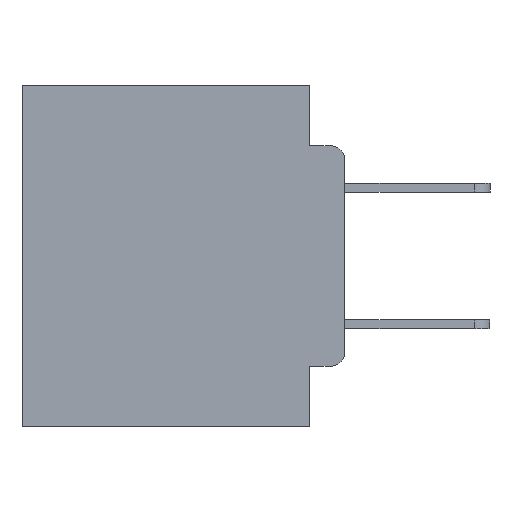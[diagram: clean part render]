
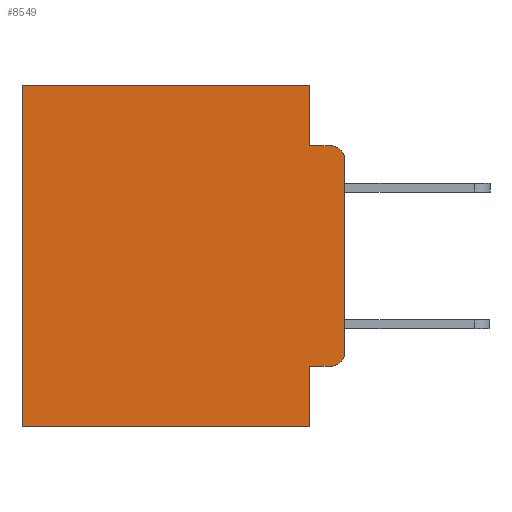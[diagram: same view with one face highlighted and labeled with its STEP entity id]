
A CAD part, left-side view. The second image highlights one B-rep face of the part: STEP entity #8549.
In plain terms, the highlighted planar face has unit normal (-1, 0, 0).
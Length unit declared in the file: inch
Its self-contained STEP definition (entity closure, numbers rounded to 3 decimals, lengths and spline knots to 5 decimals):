
#955 = DIRECTION ( 'NONE',  ( 0., 0., -1. ) ) ;
#1139 = AXIS2_PLACEMENT_3D ( 'NONE', #22405, #25187, #23031 ) ;
#1658 = CARTESIAN_POINT ( 'NONE',  ( 0.298, 0., -0.5 ) ) ;
#1908 = VERTEX_POINT ( 'NONE', #9484 ) ;
#1999 = AXIS2_PLACEMENT_3D ( 'NONE', #7386, #13831, #955 ) ;
#2071 = CARTESIAN_POINT ( 'NONE',  ( 0.298, 0., 0. ) ) ;
#2435 = EDGE_CURVE ( 'NONE', #12989, #2674, #8465, .T. ) ;
#2674 = VERTEX_POINT ( 'NONE', #13288 ) ;
#2750 = VECTOR ( 'NONE', #10493, 39.37008 ) ;
#2887 = ORIENTED_EDGE ( 'NONE', *, *, #24228, .F. ) ;
#3132 = VECTOR ( 'NONE', #14934, 39.37008 ) ;
#3242 = EDGE_CURVE ( 'NONE', #9568, #12023, #23749, .T. ) ;
#3334 = LINE ( 'NONE', #8640, #14666 ) ;
#3702 = ORIENTED_EDGE ( 'NONE', *, *, #3922, .T. ) ;
#3922 = EDGE_CURVE ( 'NONE', #1908, #19624, #14898, .T. ) ;
#3999 = VECTOR ( 'NONE', #18439, 39.37008 ) ;
#6226 = VERTEX_POINT ( 'NONE', #18835 ) ;
#6266 = VECTOR ( 'NONE', #23988, 39.37008 ) ;
#6347 = CARTESIAN_POINT ( 'NONE',  ( 0.298, 0.473, -0.5 ) ) ;
#6814 = CARTESIAN_POINT ( 'NONE',  ( 0.298, 0.051, 0. ) ) ;
#7386 = CARTESIAN_POINT ( 'NONE',  ( 0.298, 0., 0. ) ) ;
#7534 = EDGE_LOOP ( 'NONE', ( #11947, #11253, #23804, #2887, #17305, #3702, #9386, #14583, #17717, #13311 ) ) ;
#8465 = LINE ( 'NONE', #6814, #2750 ) ;
#8549 = ADVANCED_FACE ( 'NONE', ( #11725 ), #20108, .F. ) ;
#8562 = CARTESIAN_POINT ( 'NONE',  ( 0.298, 0., 0. ) ) ;
#8640 = CARTESIAN_POINT ( 'NONE',  ( 0.298, 0.051, -0.4115 ) ) ;
#8849 = LINE ( 'NONE', #1658, #3132 ) ;
#9386 = ORIENTED_EDGE ( 'NONE', *, *, #26459, .F. ) ;
#9436 = AXIS2_PLACEMENT_3D ( 'NONE', #12673, #27219, #14789 ) ;
#9484 = CARTESIAN_POINT ( 'NONE',  ( 0.298, 0.473, 0. ) ) ;
#9568 = VERTEX_POINT ( 'NONE', #25032 ) ;
#10493 = DIRECTION ( 'NONE',  ( 0., 0., -1. ) ) ;
#10741 = CARTESIAN_POINT ( 'NONE',  ( 0.298, 0.473, 0. ) ) ;
#10843 = EDGE_CURVE ( 'NONE', #9568, #13972, #24900, .T. ) ;
#10879 = EDGE_CURVE ( 'NONE', #24064, #1908, #24271, .T. ) ;
#11253 = ORIENTED_EDGE ( 'NONE', *, *, #3242, .T. ) ;
#11314 = LINE ( 'NONE', #11469, #6266 ) ;
#11469 = CARTESIAN_POINT ( 'NONE',  ( 0.298, 0.051, 0. ) ) ;
#11725 = FACE_OUTER_BOUND ( 'NONE', #7534, .T. ) ;
#11947 = ORIENTED_EDGE ( 'NONE', *, *, #10843, .F. ) ;
#12023 = VERTEX_POINT ( 'NONE', #26804 ) ;
#12257 = CIRCLE ( 'NONE', #9436, 0.02 ) ;
#12439 = CARTESIAN_POINT ( 'NONE',  ( 0.298, 0.051, -0.4115 ) ) ;
#12673 = CARTESIAN_POINT ( 'NONE',  ( 0.298, 0.02, -0.3915 ) ) ;
#12989 = VERTEX_POINT ( 'NONE', #12439 ) ;
#13288 = CARTESIAN_POINT ( 'NONE',  ( 0.298, 0.051, -0.5 ) ) ;
#13311 = ORIENTED_EDGE ( 'NONE', *, *, #20097, .T. ) ;
#13826 = VECTOR ( 'NONE', #23273, 39.37008 ) ;
#13831 = DIRECTION ( 'NONE',  ( 1., 0., 0. ) ) ;
#13972 = VERTEX_POINT ( 'NONE', #19870 ) ;
#14583 = ORIENTED_EDGE ( 'NONE', *, *, #2435, .F. ) ;
#14666 = VECTOR ( 'NONE', #25400, 39.37008 ) ;
#14789 = DIRECTION ( 'NONE',  ( 0., 0., -1. ) ) ;
#14898 = LINE ( 'NONE', #10741, #16217 ) ;
#14934 = DIRECTION ( 'NONE',  ( 0., 1., 0. ) ) ;
#16217 = VECTOR ( 'NONE', #17073, 39.37008 ) ;
#16305 = CARTESIAN_POINT ( 'NONE',  ( 0.298, 0.051, -0.0885 ) ) ;
#17073 = DIRECTION ( 'NONE',  ( 0., 0., -1. ) ) ;
#17149 = CARTESIAN_POINT ( 'NONE',  ( 0.298, 0.051, 0. ) ) ;
#17305 = ORIENTED_EDGE ( 'NONE', *, *, #10879, .T. ) ;
#17592 = VERTEX_POINT ( 'NONE', #26124 ) ;
#17717 = ORIENTED_EDGE ( 'NONE', *, *, #22864, .T. ) ;
#18439 = DIRECTION ( 'NONE',  ( 0., -1., 0. ) ) ;
#18776 = VECTOR ( 'NONE', #21323, 39.37008 ) ;
#18835 = CARTESIAN_POINT ( 'NONE',  ( 0.298, 0.02, -0.4115 ) ) ;
#19624 = VERTEX_POINT ( 'NONE', #6347 ) ;
#19870 = CARTESIAN_POINT ( 'NONE',  ( 0.298, 0., -0.3915 ) ) ;
#20097 = EDGE_CURVE ( 'NONE', #6226, #13972, #12257, .T. ) ;
#20108 = PLANE ( 'NONE',  #1999 ) ;
#20271 = LINE ( 'NONE', #16305, #3999 ) ;
#21323 = DIRECTION ( 'NONE',  ( 0., 1., 0. ) ) ;
#22405 = CARTESIAN_POINT ( 'NONE',  ( 0.298, 0.02, -0.1085 ) ) ;
#22864 = EDGE_CURVE ( 'NONE', #12989, #6226, #3334, .T. ) ;
#23031 = DIRECTION ( 'NONE',  ( 0., 0., -1. ) ) ;
#23235 = EDGE_CURVE ( 'NONE', #17592, #12023, #20271, .T. ) ;
#23273 = DIRECTION ( 'NONE',  ( 0., 0., -1. ) ) ;
#23749 = CIRCLE ( 'NONE', #1139, 0.02 ) ;
#23804 = ORIENTED_EDGE ( 'NONE', *, *, #23235, .F. ) ;
#23988 = DIRECTION ( 'NONE',  ( 0., 0., -1. ) ) ;
#24064 = VERTEX_POINT ( 'NONE', #17149 ) ;
#24228 = EDGE_CURVE ( 'NONE', #24064, #17592, #11314, .T. ) ;
#24271 = LINE ( 'NONE', #8562, #18776 ) ;
#24900 = LINE ( 'NONE', #2071, #13826 ) ;
#25032 = CARTESIAN_POINT ( 'NONE',  ( 0.298, 0., -0.1085 ) ) ;
#25187 = DIRECTION ( 'NONE',  ( -1., 0., 0. ) ) ;
#25400 = DIRECTION ( 'NONE',  ( 0., -1., 0. ) ) ;
#26124 = CARTESIAN_POINT ( 'NONE',  ( 0.298, 0.051, -0.0885 ) ) ;
#26459 = EDGE_CURVE ( 'NONE', #2674, #19624, #8849, .T. ) ;
#26804 = CARTESIAN_POINT ( 'NONE',  ( 0.298, 0.02, -0.0885 ) ) ;
#27219 = DIRECTION ( 'NONE',  ( -1., 0., 0. ) ) ;
